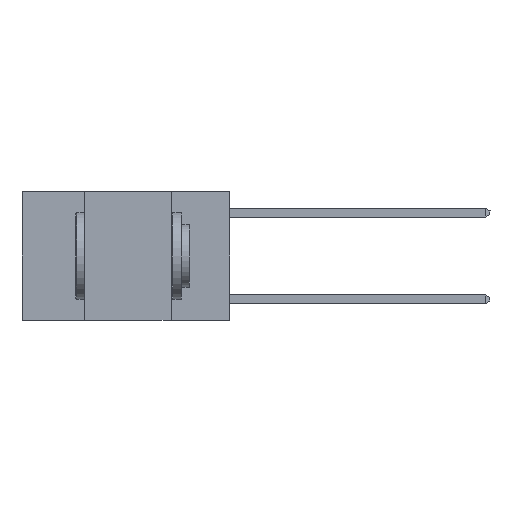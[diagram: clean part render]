
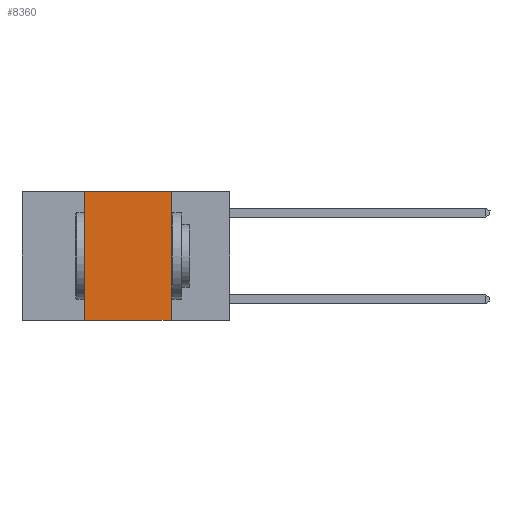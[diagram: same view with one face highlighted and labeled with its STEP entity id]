
A CAD part, left-side view. The second image highlights one B-rep face of the part: STEP entity #8360.
In plain terms, the highlighted planar face has unit normal (-1, 0, 0).
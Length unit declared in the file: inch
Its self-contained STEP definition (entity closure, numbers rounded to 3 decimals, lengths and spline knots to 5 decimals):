
#338 = VERTEX_POINT ( 'NONE', #7525 ) ;
#2103 = DIRECTION ( 'NONE',  ( 0., 0., -1. ) ) ;
#2861 = LINE ( 'NONE', #10818, #21153 ) ;
#2991 = VECTOR ( 'NONE', #2103, 39.37008 ) ;
#3426 = VERTEX_POINT ( 'NONE', #14443 ) ;
#3496 = CARTESIAN_POINT ( 'NONE',  ( 0., 0.6, 0. ) ) ;
#3819 = ORIENTED_EDGE ( 'NONE', *, *, #9707, .F. ) ;
#4648 = LINE ( 'NONE', #6383, #17387 ) ;
#5895 = DIRECTION ( 'NONE',  ( 0., 0., -1. ) ) ;
#5902 = VERTEX_POINT ( 'NONE', #6451 ) ;
#6383 = CARTESIAN_POINT ( 'NONE',  ( 0., 0.42, 0. ) ) ;
#6451 = CARTESIAN_POINT ( 'NONE',  ( 0., 0.42, -0.37 ) ) ;
#7525 = CARTESIAN_POINT ( 'NONE',  ( 0., 0.17, 0. ) ) ;
#7539 = ORIENTED_EDGE ( 'NONE', *, *, #18962, .F. ) ;
#8322 = VERTEX_POINT ( 'NONE', #15316 ) ;
#8360 = ADVANCED_FACE ( 'NONE', ( #28938 ), #20099, .F. ) ;
#8502 = DIRECTION ( 'NONE',  ( 0., -1., 0. ) ) ;
#9338 = LINE ( 'NONE', #18913, #2991 ) ;
#9707 = EDGE_CURVE ( 'NONE', #5902, #8322, #4648, .T. ) ;
#10426 = VECTOR ( 'NONE', #29725, 39.37008 ) ;
#10818 = CARTESIAN_POINT ( 'NONE',  ( 0., 0.6, -0.37 ) ) ;
#14443 = CARTESIAN_POINT ( 'NONE',  ( 0., 0.17, -0.37 ) ) ;
#14674 = ORIENTED_EDGE ( 'NONE', *, *, #20658, .T. ) ;
#15316 = CARTESIAN_POINT ( 'NONE',  ( 0., 0.42, 0. ) ) ;
#17387 = VECTOR ( 'NONE', #23122, 39.37008 ) ;
#17888 = CARTESIAN_POINT ( 'NONE',  ( 0., 0.6, 0. ) ) ;
#18913 = CARTESIAN_POINT ( 'NONE',  ( 0., 0.17, 0. ) ) ;
#18962 = EDGE_CURVE ( 'NONE', #338, #3426, #9338, .T. ) ;
#20022 = AXIS2_PLACEMENT_3D ( 'NONE', #3496, #20195, #5895 ) ;
#20099 = PLANE ( 'NONE',  #20022 ) ;
#20195 = DIRECTION ( 'NONE',  ( 1., 0., 0. ) ) ;
#20318 = EDGE_LOOP ( 'NONE', ( #7539, #20609, #3819, #14674 ) ) ;
#20609 = ORIENTED_EDGE ( 'NONE', *, *, #24955, .F. ) ;
#20658 = EDGE_CURVE ( 'NONE', #5902, #3426, #2861, .T. ) ;
#21153 = VECTOR ( 'NONE', #8502, 39.37008 ) ;
#23122 = DIRECTION ( 'NONE',  ( 0., 0., 1. ) ) ;
#24955 = EDGE_CURVE ( 'NONE', #8322, #338, #29415, .T. ) ;
#28938 = FACE_OUTER_BOUND ( 'NONE', #20318, .T. ) ;
#29415 = LINE ( 'NONE', #17888, #10426 ) ;
#29725 = DIRECTION ( 'NONE',  ( 0., -1., 0. ) ) ;
